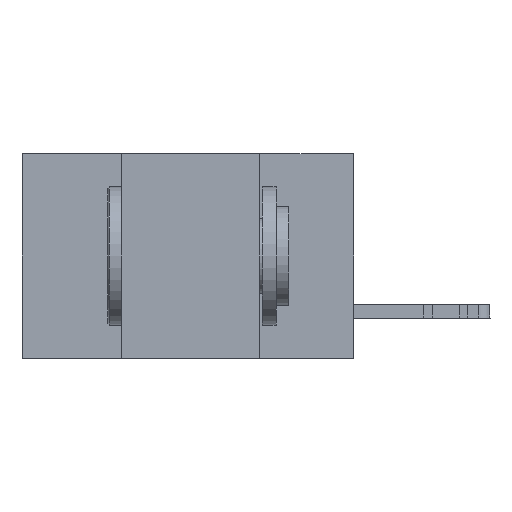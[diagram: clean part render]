
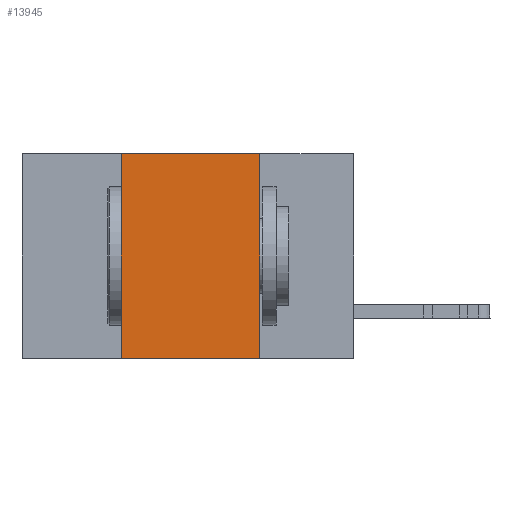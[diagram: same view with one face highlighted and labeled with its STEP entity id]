
A CAD part, left-side view. The second image highlights one B-rep face of the part: STEP entity #13945.
In plain terms, the highlighted planar face has unit normal (-1, 0, 0).
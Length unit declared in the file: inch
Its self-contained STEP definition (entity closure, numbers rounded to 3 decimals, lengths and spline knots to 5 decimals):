
#602 = LINE ( 'NONE', #2236, #29003 ) ;
#1856 = DIRECTION ( 'NONE',  ( 0., 0., -1. ) ) ;
#2236 = CARTESIAN_POINT ( 'NONE',  ( 0., 0.6, 0. ) ) ;
#3605 = ORIENTED_EDGE ( 'NONE', *, *, #26646, .T. ) ;
#5112 = CARTESIAN_POINT ( 'NONE',  ( 0., 0.42, -0.37 ) ) ;
#5261 = DIRECTION ( 'NONE',  ( 0., -1., 0. ) ) ;
#5555 = VERTEX_POINT ( 'NONE', #5112 ) ;
#6872 = DIRECTION ( 'NONE',  ( 0., 0., -1. ) ) ;
#7141 = ORIENTED_EDGE ( 'NONE', *, *, #21478, .F. ) ;
#8250 = FACE_OUTER_BOUND ( 'NONE', #15795, .T. ) ;
#9027 = VERTEX_POINT ( 'NONE', #9214 ) ;
#9214 = CARTESIAN_POINT ( 'NONE',  ( 0., 0.42, 0. ) ) ;
#9293 = EDGE_CURVE ( 'NONE', #42534, #39613, #37073, .T. ) ;
#9976 = VECTOR ( 'NONE', #21186, 39.37008 ) ;
#10485 = PLANE ( 'NONE',  #14316 ) ;
#13799 = DIRECTION ( 'NONE',  ( 1., 0., 0. ) ) ;
#13945 = ADVANCED_FACE ( 'NONE', ( #8250 ), #10485, .F. ) ;
#14316 = AXIS2_PLACEMENT_3D ( 'NONE', #30123, #13799, #6872 ) ;
#15795 = EDGE_LOOP ( 'NONE', ( #32611, #25841, #7141, #3605 ) ) ;
#17162 = LINE ( 'NONE', #29908, #32693 ) ;
#17871 = CARTESIAN_POINT ( 'NONE',  ( 0., 0.42, 0. ) ) ;
#18675 = CARTESIAN_POINT ( 'NONE',  ( 0., 0.17, -0.37 ) ) ;
#21186 = DIRECTION ( 'NONE',  ( 0., 0., 1. ) ) ;
#21478 = EDGE_CURVE ( 'NONE', #5555, #9027, #33778, .T. ) ;
#22163 = EDGE_CURVE ( 'NONE', #9027, #42534, #602, .T. ) ;
#22972 = DIRECTION ( 'NONE',  ( 0., -1., 0. ) ) ;
#24665 = VECTOR ( 'NONE', #1856, 39.37008 ) ;
#25841 = ORIENTED_EDGE ( 'NONE', *, *, #22163, .F. ) ;
#26646 = EDGE_CURVE ( 'NONE', #5555, #39613, #17162, .T. ) ;
#29003 = VECTOR ( 'NONE', #5261, 39.37008 ) ;
#29908 = CARTESIAN_POINT ( 'NONE',  ( 0., 0.6, -0.37 ) ) ;
#30123 = CARTESIAN_POINT ( 'NONE',  ( 0., 0.6, 0. ) ) ;
#32611 = ORIENTED_EDGE ( 'NONE', *, *, #9293, .F. ) ;
#32693 = VECTOR ( 'NONE', #22972, 39.37008 ) ;
#33778 = LINE ( 'NONE', #17871, #9976 ) ;
#37073 = LINE ( 'NONE', #38090, #24665 ) ;
#37763 = CARTESIAN_POINT ( 'NONE',  ( 0., 0.17, 0. ) ) ;
#38090 = CARTESIAN_POINT ( 'NONE',  ( 0., 0.17, 0. ) ) ;
#39613 = VERTEX_POINT ( 'NONE', #18675 ) ;
#42534 = VERTEX_POINT ( 'NONE', #37763 ) ;
